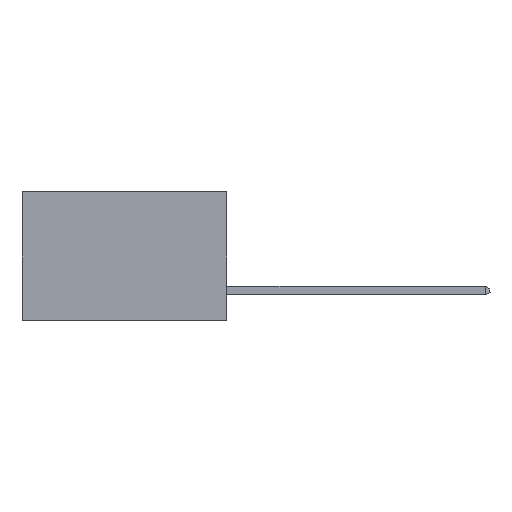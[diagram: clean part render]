
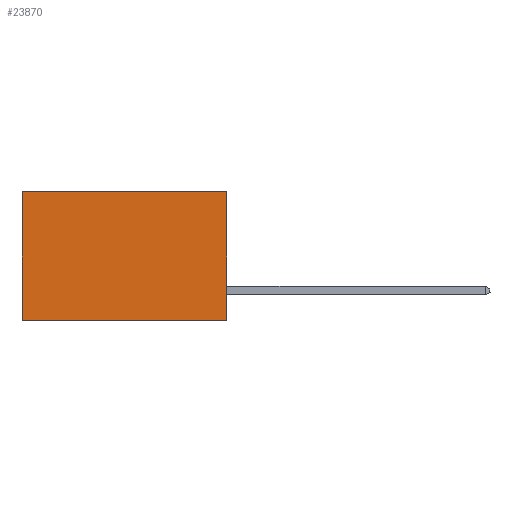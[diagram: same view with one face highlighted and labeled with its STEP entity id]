
A CAD part, left-side view. The second image highlights one B-rep face of the part: STEP entity #23870.
In plain terms, the highlighted planar face has unit normal (-1, 0, 0).
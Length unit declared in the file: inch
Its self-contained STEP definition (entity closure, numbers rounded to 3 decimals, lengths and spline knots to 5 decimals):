
#473 = VECTOR ( 'NONE', #16227, 39.37008 ) ;
#2021 = CARTESIAN_POINT ( 'NONE',  ( 0.277, 0.59, -0.37 ) ) ;
#3007 = ORIENTED_EDGE ( 'NONE', *, *, #8011, .T. ) ;
#3420 = VECTOR ( 'NONE', #4407, 39.37008 ) ;
#4375 = EDGE_CURVE ( 'NONE', #17407, #27670, #4601, .T. ) ;
#4407 = DIRECTION ( 'NONE',  ( 0., 0., -1. ) ) ;
#4601 = LINE ( 'NONE', #10231, #22974 ) ;
#5579 = EDGE_LOOP ( 'NONE', ( #7776, #16829, #13083, #3007 ) ) ;
#6449 = CARTESIAN_POINT ( 'NONE',  ( 0.277, 0.59, -0.37 ) ) ;
#7776 = ORIENTED_EDGE ( 'NONE', *, *, #21709, .T. ) ;
#8011 = EDGE_CURVE ( 'NONE', #17407, #25281, #30653, .T. ) ;
#8245 = CARTESIAN_POINT ( 'NONE',  ( 0.277, 0., -0.37 ) ) ;
#10231 = CARTESIAN_POINT ( 'NONE',  ( 0.277, 0., -0.37 ) ) ;
#10628 = DIRECTION ( 'NONE',  ( 0., 1., 0. ) ) ;
#10675 = CARTESIAN_POINT ( 'NONE',  ( 0.277, 0.59, 0. ) ) ;
#11870 = LINE ( 'NONE', #8245, #17497 ) ;
#12463 = EDGE_CURVE ( 'NONE', #27670, #26085, #11870, .T. ) ;
#13083 = ORIENTED_EDGE ( 'NONE', *, *, #4375, .F. ) ;
#15221 = DIRECTION ( 'NONE',  ( 0., 0., -1. ) ) ;
#15804 = CARTESIAN_POINT ( 'NONE',  ( 0.277, 0., 0. ) ) ;
#16161 = LINE ( 'NONE', #2021, #3420 ) ;
#16227 = DIRECTION ( 'NONE',  ( 0., 1., 0. ) ) ;
#16829 = ORIENTED_EDGE ( 'NONE', *, *, #12463, .F. ) ;
#17407 = VERTEX_POINT ( 'NONE', #26021 ) ;
#17497 = VECTOR ( 'NONE', #10628, 39.37008 ) ;
#18162 = DIRECTION ( 'NONE',  ( 0., 0., -1. ) ) ;
#19947 = CARTESIAN_POINT ( 'NONE',  ( 0.277, 0., -0.37 ) ) ;
#21709 = EDGE_CURVE ( 'NONE', #25281, #26085, #16161, .T. ) ;
#22974 = VECTOR ( 'NONE', #18162, 39.37008 ) ;
#23111 = FACE_OUTER_BOUND ( 'NONE', #5579, .T. ) ;
#23870 = ADVANCED_FACE ( 'NONE', ( #23111 ), #24729, .F. ) ;
#24729 = PLANE ( 'NONE',  #27158 ) ;
#25281 = VERTEX_POINT ( 'NONE', #10675 ) ;
#26021 = CARTESIAN_POINT ( 'NONE',  ( 0.277, 0., 0. ) ) ;
#26085 = VERTEX_POINT ( 'NONE', #6449 ) ;
#27158 = AXIS2_PLACEMENT_3D ( 'NONE', #19947, #29408, #15221 ) ;
#27670 = VERTEX_POINT ( 'NONE', #28559 ) ;
#28559 = CARTESIAN_POINT ( 'NONE',  ( 0.277, 0., -0.37 ) ) ;
#29408 = DIRECTION ( 'NONE',  ( 1., 0., 0. ) ) ;
#30653 = LINE ( 'NONE', #15804, #473 ) ;
